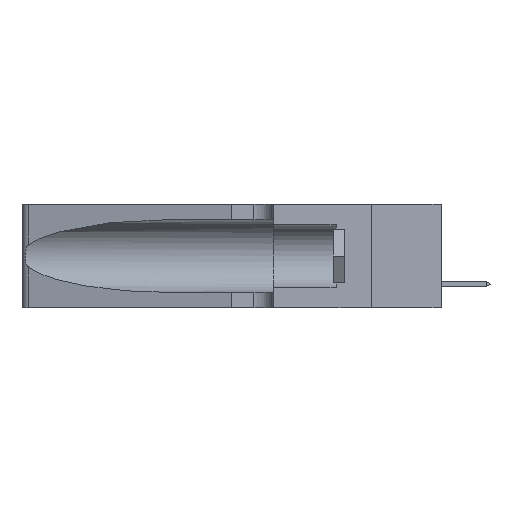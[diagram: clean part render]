
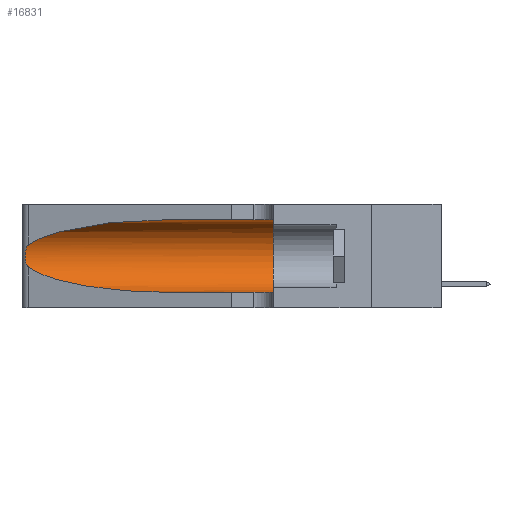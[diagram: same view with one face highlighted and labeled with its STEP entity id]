
A CAD part, left-side view. The second image highlights one B-rep face of the part: STEP entity #16831.
In plain terms, the highlighted cylindrical face has radius 3.308 mm (diameter 6.617 mm), a partial arc.
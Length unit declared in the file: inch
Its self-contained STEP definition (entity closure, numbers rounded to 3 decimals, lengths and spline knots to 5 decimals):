
#176 = CARTESIAN_POINT ( 'NONE',  ( 0.18966, 0.96281, 0.05475 ) ) ;
#216 = ORIENTED_EDGE ( 'NONE', *, *, #17338, .F. ) ;
#319 = ORIENTED_EDGE ( 'NONE', *, *, #19137, .T. ) ;
#418 = CARTESIAN_POINT ( 'NONE',  ( 0.1305, 0.72297, 0.05475 ) ) ;
#1399 = CARTESIAN_POINT ( 'NONE',  ( 0.26018, 1.23835, 0.19895 ) ) ;
#1813 = CARTESIAN_POINT ( 'NONE',  ( 0.25487, 1.22718, 0.14631 ) ) ;
#2563 = CARTESIAN_POINT ( 'NONE',  ( 0.1305, 0.72297, 0.05475 ) ) ;
#2931 = VERTEX_POINT ( 'NONE', #19186 ) ;
#3911 = CARTESIAN_POINT ( 'NONE',  ( 0.25639, 1.23186, 0.15144 ) ) ;
#4385 = CARTESIAN_POINT ( 'NONE',  ( 0.2373, 1.15595, 0.28018 ) ) ;
#4807 = DIRECTION ( 'NONE',  ( 0., -1., 0. ) ) ;
#5181 = ORIENTED_EDGE ( 'NONE', *, *, #22960, .T. ) ;
#5320 = CARTESIAN_POINT ( 'NONE',  ( 0.1305, 0.35, 0.05475 ) ) ;
#5675 = DIRECTION ( 'NONE',  ( 0., -1., 0. ) ) ;
#6200 = CARTESIAN_POINT ( 'NONE',  ( 0.25856, 1.23593, 0.16098 ) ) ;
#6615 = CARTESIAN_POINT ( 'NONE',  ( 0.1305, 0.35, 0.31525 ) ) ;
#7184 = CIRCLE ( 'NONE', #16406, 0.13025 ) ;
#7522 = VECTOR ( 'NONE', #12759, 39.37008 ) ;
#8250 = B_SPLINE_CURVE_WITH_KNOTS ( 'NONE', 3,
 ( #22749, #30109, #15880, #27380, #15683, #1399, #18155, #18047, #20464, #6200, #8617, #3911, #16084, #1813 ),
 .UNSPECIFIED., .F., .F.,
 ( 4, 2, 2, 2, 2, 2, 4 ),
 ( 0., 0.00027, 0.00053, 0.00107, 0.0016, 0.00187, 0.00214 ),
 .UNSPECIFIED. ) ;
#8617 = CARTESIAN_POINT ( 'NONE',  ( 0.25789, 1.23486, 0.15765 ) ) ;
#8680 = CARTESIAN_POINT ( 'NONE',  ( 0.1305, 0.72297, 0.31525 ) ) ;
#8833 = VERTEX_POINT ( 'NONE', #19277 ) ;
#9807 = CARTESIAN_POINT ( 'NONE',  ( 0.1305, 1.61858, 0.31525 ) ) ;
#10074 = CARTESIAN_POINT ( 'NONE',  ( 0.2373, 1.15595, 0.08982 ) ) ;
#10609 = LINE ( 'NONE', #9807, #29562 ) ;
#12759 = DIRECTION ( 'NONE',  ( 0., -1., 0. ) ) ;
#13229 = EDGE_CURVE ( 'NONE', #13879, #2931, #14280, .T. ) ;
#13337 = ORIENTED_EDGE ( 'NONE', *, *, #18260, .F. ) ;
#13879 = VERTEX_POINT ( 'NONE', #28595 ) ;
#14280 =( BOUNDED_CURVE ( )  B_SPLINE_CURVE ( 3, ( #8680, #30361, #4385, #16325 ),
 .UNSPECIFIED., .F., .T. ) 
 B_SPLINE_CURVE_WITH_KNOTS ( ( 4, 4 ),
 ( 1.5708, 2.84003 ),
 .UNSPECIFIED. ) 
 CURVE ( )  GEOMETRIC_REPRESENTATION_ITEM ( )  RATIONAL_B_SPLINE_CURVE ( ( 1., 0.87, 0.87, 1. ) ) 
 REPRESENTATION_ITEM ( '' )  );
#14352 = CYLINDRICAL_SURFACE ( 'NONE', #27324, 0.13025 ) ;
#14418 = CARTESIAN_POINT ( 'NONE',  ( 0.25487, 1.22718, 0.14631 ) ) ;
#15465 = DIRECTION ( 'NONE',  ( 0., 0., -1. ) ) ;
#15683 = CARTESIAN_POINT ( 'NONE',  ( 0.25854, 1.2359, 0.20912 ) ) ;
#15880 = CARTESIAN_POINT ( 'NONE',  ( 0.25639, 1.23184, 0.21858 ) ) ;
#16084 = CARTESIAN_POINT ( 'NONE',  ( 0.25555, 1.22993, 0.14849 ) ) ;
#16209 = VERTEX_POINT ( 'NONE', #6615 ) ;
#16255 = CARTESIAN_POINT ( 'NONE',  ( 0.1305, 0.35, 0.185 ) ) ;
#16325 = CARTESIAN_POINT ( 'NONE',  ( 0.25487, 1.22718, 0.22369 ) ) ;
#16406 = AXIS2_PLACEMENT_3D ( 'NONE', #16255, #18137, #25300 ) ;
#16831 = ADVANCED_FACE ( 'NONE', ( #30351 ), #14352, .F. ) ;
#16967 =( BOUNDED_CURVE ( )  B_SPLINE_CURVE ( 3, ( #14418, #10074, #176, #2563 ),
 .UNSPECIFIED., .F., .F. ) 
 B_SPLINE_CURVE_WITH_KNOTS ( ( 4, 4 ),
 ( 3.44316, 4.71239 ),
 .UNSPECIFIED. ) 
 CURVE ( )  GEOMETRIC_REPRESENTATION_ITEM ( )  RATIONAL_B_SPLINE_CURVE ( ( 1., 0.87, 0.87, 1. ) ) 
 REPRESENTATION_ITEM ( '' )  );
#17338 = EDGE_CURVE ( 'NONE', #13879, #16209, #10609, .T. ) ;
#18047 = CARTESIAN_POINT ( 'NONE',  ( 0.26075, 1.23896, 0.178 ) ) ;
#18137 = DIRECTION ( 'NONE',  ( 0., 1., 0. ) ) ;
#18155 = CARTESIAN_POINT ( 'NONE',  ( 0.26075, 1.23896, 0.19203 ) ) ;
#18255 = ORIENTED_EDGE ( 'NONE', *, *, #13229, .T. ) ;
#18260 = EDGE_CURVE ( 'NONE', #16209, #24178, #7184, .T. ) ;
#19137 = EDGE_CURVE ( 'NONE', #24642, #24178, #20162, .T. ) ;
#19186 = CARTESIAN_POINT ( 'NONE',  ( 0.25487, 1.22718, 0.22369 ) ) ;
#19277 = CARTESIAN_POINT ( 'NONE',  ( 0.25487, 1.22718, 0.14631 ) ) ;
#20162 = LINE ( 'NONE', #29511, #7522 ) ;
#20343 = CARTESIAN_POINT ( 'NONE',  ( 0.1305, 1.61858, 0.185 ) ) ;
#20464 = CARTESIAN_POINT ( 'NONE',  ( 0.26017, 1.23833, 0.17102 ) ) ;
#21010 = EDGE_CURVE ( 'NONE', #8833, #24642, #16967, .T. ) ;
#22749 = CARTESIAN_POINT ( 'NONE',  ( 0.25487, 1.22718, 0.22369 ) ) ;
#22960 = EDGE_CURVE ( 'NONE', #2931, #8833, #8250, .T. ) ;
#24178 = VERTEX_POINT ( 'NONE', #5320 ) ;
#24642 = VERTEX_POINT ( 'NONE', #418 ) ;
#24819 = ORIENTED_EDGE ( 'NONE', *, *, #21010, .T. ) ;
#25300 = DIRECTION ( 'NONE',  ( 0., 0., 1. ) ) ;
#26447 = EDGE_LOOP ( 'NONE', ( #18255, #5181, #24819, #319, #13337, #216 ) ) ;
#27324 = AXIS2_PLACEMENT_3D ( 'NONE', #20343, #5675, #15465 ) ;
#27380 = CARTESIAN_POINT ( 'NONE',  ( 0.25787, 1.23484, 0.2124 ) ) ;
#28595 = CARTESIAN_POINT ( 'NONE',  ( 0.1305, 0.72297, 0.31525 ) ) ;
#29511 = CARTESIAN_POINT ( 'NONE',  ( 0.1305, 1.61858, 0.05475 ) ) ;
#29562 = VECTOR ( 'NONE', #4807, 39.37008 ) ;
#30109 = CARTESIAN_POINT ( 'NONE',  ( 0.25555, 1.22994, 0.2215 ) ) ;
#30351 = FACE_OUTER_BOUND ( 'NONE', #26447, .T. ) ;
#30361 = CARTESIAN_POINT ( 'NONE',  ( 0.18966, 0.96281, 0.31525 ) ) ;
